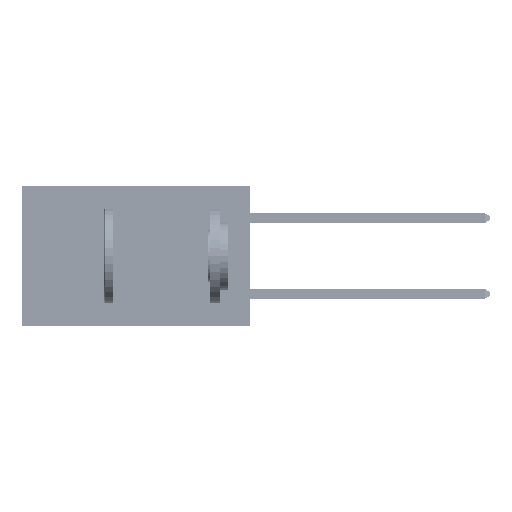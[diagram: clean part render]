
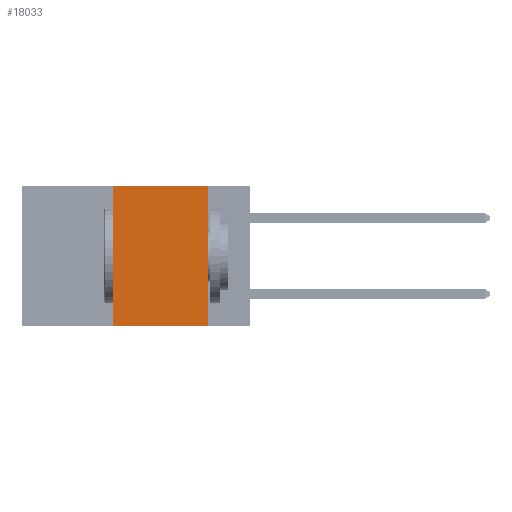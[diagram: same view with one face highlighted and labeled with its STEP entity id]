
A CAD part, left-side view. The second image highlights one B-rep face of the part: STEP entity #18033.
In plain terms, the highlighted planar face has unit normal (-1, 0, 0).
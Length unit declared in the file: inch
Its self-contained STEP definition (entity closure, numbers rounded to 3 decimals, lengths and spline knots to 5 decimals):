
#1431 = VECTOR ( 'NONE', #23649, 39.37008 ) ;
#2595 = CARTESIAN_POINT ( 'NONE',  ( 0., 0.6, -0.37 ) ) ;
#5894 = CARTESIAN_POINT ( 'NONE',  ( 0., 0.11, -0.37 ) ) ;
#6523 = DIRECTION ( 'NONE',  ( 0., 0., 1. ) ) ;
#10688 = CARTESIAN_POINT ( 'NONE',  ( 0., 0.6, 0. ) ) ;
#11228 = LINE ( 'NONE', #2595, #12468 ) ;
#11687 = EDGE_CURVE ( 'NONE', #33815, #42500, #40039, .T. ) ;
#12468 = VECTOR ( 'NONE', #49647, 39.37008 ) ;
#15627 = LINE ( 'NONE', #10688, #48139 ) ;
#17408 = FACE_OUTER_BOUND ( 'NONE', #46878, .T. ) ;
#18033 = ADVANCED_FACE ( 'NONE', ( #17408 ), #37263, .F. ) ;
#18465 = CARTESIAN_POINT ( 'NONE',  ( 0., 0.11, 0. ) ) ;
#18475 = VERTEX_POINT ( 'NONE', #40146 ) ;
#21654 = CARTESIAN_POINT ( 'NONE',  ( 0., 0.6, 0. ) ) ;
#23649 = DIRECTION ( 'NONE',  ( 0., 0., -1. ) ) ;
#24714 = CARTESIAN_POINT ( 'NONE',  ( 0., 0.36, -0.37 ) ) ;
#27036 = ORIENTED_EDGE ( 'NONE', *, *, #11687, .F. ) ;
#29109 = CARTESIAN_POINT ( 'NONE',  ( 0., 0.36, 0. ) ) ;
#30799 = ORIENTED_EDGE ( 'NONE', *, *, #41048, .F. ) ;
#31106 = ORIENTED_EDGE ( 'NONE', *, *, #50576, .T. ) ;
#33768 = EDGE_CURVE ( 'NONE', #45559, #18475, #47463, .T. ) ;
#33815 = VERTEX_POINT ( 'NONE', #18465 ) ;
#33954 = CARTESIAN_POINT ( 'NONE',  ( 0., 0.11, 0. ) ) ;
#36410 = VECTOR ( 'NONE', #6523, 39.37008 ) ;
#37263 = PLANE ( 'NONE',  #43583 ) ;
#37430 = DIRECTION ( 'NONE',  ( 0., 0., -1. ) ) ;
#40039 = LINE ( 'NONE', #33954, #1431 ) ;
#40146 = CARTESIAN_POINT ( 'NONE',  ( 0., 0.36, 0. ) ) ;
#40686 = ORIENTED_EDGE ( 'NONE', *, *, #33768, .F. ) ;
#41048 = EDGE_CURVE ( 'NONE', #18475, #33815, #15627, .T. ) ;
#42500 = VERTEX_POINT ( 'NONE', #5894 ) ;
#43583 = AXIS2_PLACEMENT_3D ( 'NONE', #21654, #49069, #37430 ) ;
#45559 = VERTEX_POINT ( 'NONE', #24714 ) ;
#45792 = DIRECTION ( 'NONE',  ( 0., -1., 0. ) ) ;
#46878 = EDGE_LOOP ( 'NONE', ( #27036, #30799, #40686, #31106 ) ) ;
#47463 = LINE ( 'NONE', #29109, #36410 ) ;
#48139 = VECTOR ( 'NONE', #45792, 39.37008 ) ;
#49069 = DIRECTION ( 'NONE',  ( 1., 0., 0. ) ) ;
#49647 = DIRECTION ( 'NONE',  ( 0., -1., 0. ) ) ;
#50576 = EDGE_CURVE ( 'NONE', #45559, #42500, #11228, .T. ) ;
